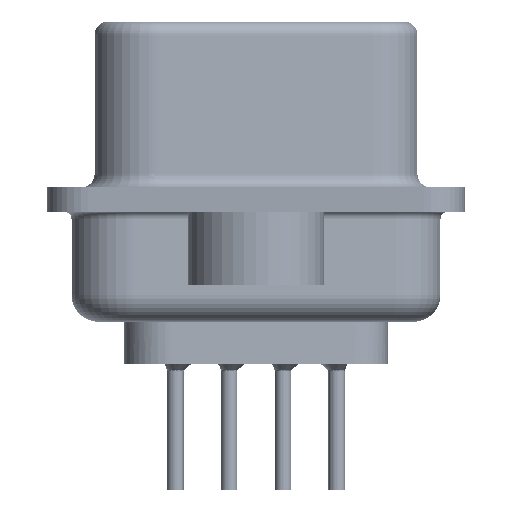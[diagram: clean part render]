
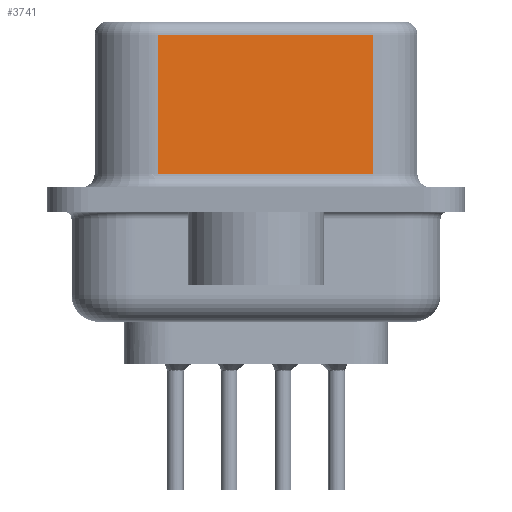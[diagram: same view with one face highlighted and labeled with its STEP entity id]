
A CAD part, left-side view. The second image highlights one B-rep face of the part: STEP entity #3741.
In plain terms, the highlighted planar face has unit normal (-0.985, -0.174, 0).
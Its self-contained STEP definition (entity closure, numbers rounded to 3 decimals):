
#176 = VERTEX_POINT ( 'NONE', #30159 ) ;
#310 = EDGE_CURVE ( 'NONE', #22352, #176, #10302, .T. ) ;
#1020 = PLANE ( 'NONE',  #20926 ) ;
#1522 = EDGE_LOOP ( 'NONE', ( #28030, #21171, #42878, #17176 ) ) ;
#3741 = ADVANCED_FACE ( 'NONE', ( #4798 ), #1020, .F. ) ;
#4394 = LINE ( 'NONE', #15033, #13684 ) ;
#4798 = FACE_OUTER_BOUND ( 'NONE', #1522, .T. ) ;
#6077 = VERTEX_POINT ( 'NONE', #10114 ) ;
#9823 = DIRECTION ( 'NONE',  ( -0.174, 0.985, 0. ) ) ;
#10114 = CARTESIAN_POINT ( 'NONE',  ( 5.128, -4.297, 0.95 ) ) ;
#10302 = LINE ( 'NONE', #16896, #10308 ) ;
#10308 = VECTOR ( 'NONE', #9823, 1000. ) ;
#11158 = EDGE_CURVE ( 'NONE', #12844, #6077, #35064, .T. ) ;
#12844 = VERTEX_POINT ( 'NONE', #15476 ) ;
#13684 = VECTOR ( 'NONE', #28985, 1000. ) ;
#15033 = CARTESIAN_POINT ( 'NONE',  ( 5.128, -4.297, 6.57 ) ) ;
#15476 = CARTESIAN_POINT ( 'NONE',  ( 3.735, 3.603, 0.95 ) ) ;
#16896 = CARTESIAN_POINT ( 'NONE',  ( 5.128, -4.297, 6.07 ) ) ;
#17176 = ORIENTED_EDGE ( 'NONE', *, *, #11158, .T. ) ;
#17298 = DIRECTION ( 'NONE',  ( 0.174, -0.985, 0. ) ) ;
#17981 = EDGE_CURVE ( 'NONE', #176, #12844, #24132, .T. ) ;
#18374 = DIRECTION ( 'NONE',  ( 0., 0., -1. ) ) ;
#19226 = CARTESIAN_POINT ( 'NONE',  ( 5.128, -4.297, 6.57 ) ) ;
#19673 = DIRECTION ( 'NONE',  ( 0.985, 0.174, 0. ) ) ;
#20926 = AXIS2_PLACEMENT_3D ( 'NONE', #19226, #19673, #34107 ) ;
#21171 = ORIENTED_EDGE ( 'NONE', *, *, #310, .T. ) ;
#22352 = VERTEX_POINT ( 'NONE', #34709 ) ;
#24132 = LINE ( 'NONE', #32142, #45143 ) ;
#25112 = CARTESIAN_POINT ( 'NONE',  ( 5.128, -4.297, 0.95 ) ) ;
#27250 = EDGE_CURVE ( 'NONE', #22352, #6077, #4394, .T. ) ;
#28030 = ORIENTED_EDGE ( 'NONE', *, *, #27250, .F. ) ;
#28985 = DIRECTION ( 'NONE',  ( 0., 0., -1. ) ) ;
#30159 = CARTESIAN_POINT ( 'NONE',  ( 3.735, 3.603, 6.07 ) ) ;
#32142 = CARTESIAN_POINT ( 'NONE',  ( 3.735, 3.603, 6.57 ) ) ;
#34107 = DIRECTION ( 'NONE',  ( -0.174, 0.985, 0. ) ) ;
#34709 = CARTESIAN_POINT ( 'NONE',  ( 5.128, -4.297, 6.07 ) ) ;
#35064 = LINE ( 'NONE', #25112, #38049 ) ;
#38049 = VECTOR ( 'NONE', #17298, 1000. ) ;
#42878 = ORIENTED_EDGE ( 'NONE', *, *, #17981, .T. ) ;
#45143 = VECTOR ( 'NONE', #18374, 1000. ) ;
